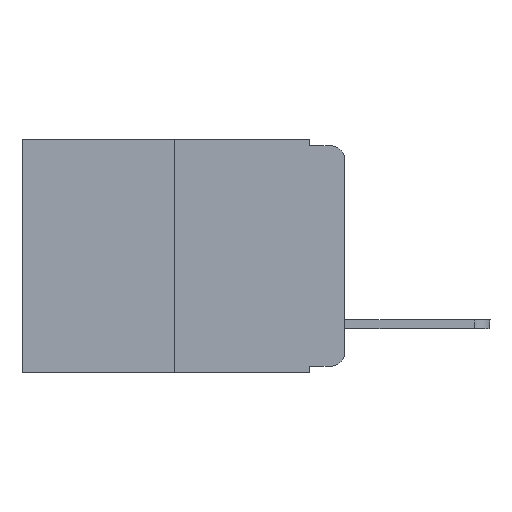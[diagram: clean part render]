
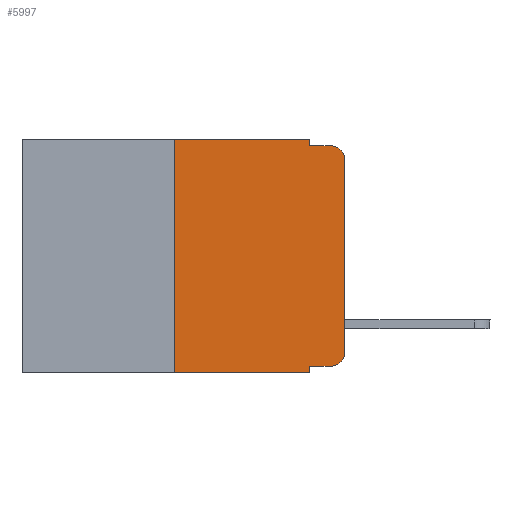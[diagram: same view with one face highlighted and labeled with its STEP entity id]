
A CAD part, left-side view. The second image highlights one B-rep face of the part: STEP entity #5997.
In plain terms, the highlighted planar face has unit normal (-1, 0, 0).
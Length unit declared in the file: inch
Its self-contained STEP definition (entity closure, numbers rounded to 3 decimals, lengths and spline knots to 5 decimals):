
#71 = EDGE_LOOP ( 'NONE', ( #4447, #2612, #941, #431, #14906, #1251, #9153, #8922, #10786, #6475 ) ) ;
#115 = LINE ( 'NONE', #4852, #1007 ) ;
#431 = ORIENTED_EDGE ( 'NONE', *, *, #6474, .F. ) ;
#554 = CARTESIAN_POINT ( 'NONE',  ( 0., 0., 0. ) ) ;
#941 = ORIENTED_EDGE ( 'NONE', *, *, #1048, .F. ) ;
#1007 = VECTOR ( 'NONE', #3630, 39.37008 ) ;
#1048 = EDGE_CURVE ( 'NONE', #14883, #9292, #13032, .T. ) ;
#1094 = VERTEX_POINT ( 'NONE', #13824 ) ;
#1161 = EDGE_CURVE ( 'NONE', #6548, #1186, #4640, .T. ) ;
#1186 = VERTEX_POINT ( 'NONE', #9371 ) ;
#1251 = ORIENTED_EDGE ( 'NONE', *, *, #9533, .F. ) ;
#1529 = VECTOR ( 'NONE', #3277, 39.37008 ) ;
#1835 = LINE ( 'NONE', #14766, #11890 ) ;
#2115 = CARTESIAN_POINT ( 'NONE',  ( 0., 0., -0.313 ) ) ;
#2176 = CARTESIAN_POINT ( 'NONE',  ( 0., 0.051, 0. ) ) ;
#2202 = DIRECTION ( 'NONE',  ( 1., 0., 0. ) ) ;
#2219 = AXIS2_PLACEMENT_3D ( 'NONE', #8562, #2857, #4014 ) ;
#2291 = CARTESIAN_POINT ( 'NONE',  ( 0., 0.051, -0.01 ) ) ;
#2612 = ORIENTED_EDGE ( 'NONE', *, *, #7987, .T. ) ;
#2713 = LINE ( 'NONE', #3019, #14389 ) ;
#2857 = DIRECTION ( 'NONE',  ( -1., 0., 0. ) ) ;
#2916 = DIRECTION ( 'NONE',  ( 0., 0., 1. ) ) ;
#3019 = CARTESIAN_POINT ( 'NONE',  ( 0., 0.473, 0. ) ) ;
#3277 = DIRECTION ( 'NONE',  ( 0., -1., 0. ) ) ;
#3625 = CARTESIAN_POINT ( 'NONE',  ( 0., 0.051, 0. ) ) ;
#3630 = DIRECTION ( 'NONE',  ( 0., 0., 1. ) ) ;
#3824 = VECTOR ( 'NONE', #15076, 39.37008 ) ;
#4014 = DIRECTION ( 'NONE',  ( 0., 0., -1. ) ) ;
#4122 = CIRCLE ( 'NONE', #5541, 0.02 ) ;
#4413 = DIRECTION ( 'NONE',  ( 0., -1., 0. ) ) ;
#4447 = ORIENTED_EDGE ( 'NONE', *, *, #13112, .T. ) ;
#4640 = LINE ( 'NONE', #10263, #1529 ) ;
#4852 = CARTESIAN_POINT ( 'NONE',  ( 0., 0.25, 0. ) ) ;
#5175 = VECTOR ( 'NONE', #4413, 39.37008 ) ;
#5195 = CARTESIAN_POINT ( 'NONE',  ( 0., 0.25, 0. ) ) ;
#5541 = AXIS2_PLACEMENT_3D ( 'NONE', #6458, #14617, #13501 ) ;
#5729 = CARTESIAN_POINT ( 'NONE',  ( 0., 0.473, -0.343 ) ) ;
#5767 = CARTESIAN_POINT ( 'NONE',  ( 0., 0.473, 0. ) ) ;
#5997 = ADVANCED_FACE ( 'NONE', ( #12350 ), #6975, .F. ) ;
#6458 = CARTESIAN_POINT ( 'NONE',  ( 0., 0.02, -0.313 ) ) ;
#6474 = EDGE_CURVE ( 'NONE', #11374, #14883, #1835, .T. ) ;
#6475 = ORIENTED_EDGE ( 'NONE', *, *, #8776, .T. ) ;
#6548 = VERTEX_POINT ( 'NONE', #14654 ) ;
#6975 = PLANE ( 'NONE',  #9630 ) ;
#7587 = DIRECTION ( 'NONE',  ( 0., 0., -1. ) ) ;
#7809 = EDGE_CURVE ( 'NONE', #1094, #10019, #7991, .T. ) ;
#7987 = EDGE_CURVE ( 'NONE', #13256, #9292, #10720, .T. ) ;
#7991 = LINE ( 'NONE', #5729, #11484 ) ;
#8155 = VERTEX_POINT ( 'NONE', #5195 ) ;
#8485 = CARTESIAN_POINT ( 'NONE',  ( 0., 0., -0.03 ) ) ;
#8562 = CARTESIAN_POINT ( 'NONE',  ( 0., 0.02, -0.03 ) ) ;
#8776 = EDGE_CURVE ( 'NONE', #1186, #10835, #4122, .T. ) ;
#8922 = ORIENTED_EDGE ( 'NONE', *, *, #12785, .F. ) ;
#9153 = ORIENTED_EDGE ( 'NONE', *, *, #7809, .T. ) ;
#9292 = VERTEX_POINT ( 'NONE', #9966 ) ;
#9371 = CARTESIAN_POINT ( 'NONE',  ( 0., 0.02, -0.333 ) ) ;
#9533 = EDGE_CURVE ( 'NONE', #1094, #8155, #115, .T. ) ;
#9630 = AXIS2_PLACEMENT_3D ( 'NONE', #5767, #2202, #12869 ) ;
#9966 = CARTESIAN_POINT ( 'NONE',  ( 0., 0.02, -0.01 ) ) ;
#10019 = VERTEX_POINT ( 'NONE', #14010 ) ;
#10263 = CARTESIAN_POINT ( 'NONE',  ( 0., 0.051, -0.333 ) ) ;
#10720 = CIRCLE ( 'NONE', #2219, 0.02 ) ;
#10751 = CARTESIAN_POINT ( 'NONE',  ( 0., 0.051, -0.01 ) ) ;
#10786 = ORIENTED_EDGE ( 'NONE', *, *, #1161, .T. ) ;
#10835 = VERTEX_POINT ( 'NONE', #2115 ) ;
#11183 = DIRECTION ( 'NONE',  ( 0., -1., 0. ) ) ;
#11374 = VERTEX_POINT ( 'NONE', #3625 ) ;
#11484 = VECTOR ( 'NONE', #15119, 39.37008 ) ;
#11890 = VECTOR ( 'NONE', #7587, 39.37008 ) ;
#12350 = FACE_OUTER_BOUND ( 'NONE', #71, .T. ) ;
#12785 = EDGE_CURVE ( 'NONE', #6548, #10019, #14781, .T. ) ;
#12869 = DIRECTION ( 'NONE',  ( 0., 0., -1. ) ) ;
#13032 = LINE ( 'NONE', #2291, #5175 ) ;
#13112 = EDGE_CURVE ( 'NONE', #10835, #13256, #13883, .T. ) ;
#13256 = VERTEX_POINT ( 'NONE', #8485 ) ;
#13501 = DIRECTION ( 'NONE',  ( 0., 0., -1. ) ) ;
#13824 = CARTESIAN_POINT ( 'NONE',  ( 0., 0.25, -0.343 ) ) ;
#13883 = LINE ( 'NONE', #554, #14961 ) ;
#13915 = EDGE_CURVE ( 'NONE', #8155, #11374, #2713, .T. ) ;
#14010 = CARTESIAN_POINT ( 'NONE',  ( 0., 0.051, -0.343 ) ) ;
#14389 = VECTOR ( 'NONE', #11183, 39.37008 ) ;
#14617 = DIRECTION ( 'NONE',  ( -1., 0., 0. ) ) ;
#14654 = CARTESIAN_POINT ( 'NONE',  ( 0., 0.051, -0.333 ) ) ;
#14766 = CARTESIAN_POINT ( 'NONE',  ( 0., 0.051, 0. ) ) ;
#14781 = LINE ( 'NONE', #2176, #3824 ) ;
#14883 = VERTEX_POINT ( 'NONE', #10751 ) ;
#14906 = ORIENTED_EDGE ( 'NONE', *, *, #13915, .F. ) ;
#14961 = VECTOR ( 'NONE', #2916, 39.37008 ) ;
#15076 = DIRECTION ( 'NONE',  ( 0., 0., -1. ) ) ;
#15119 = DIRECTION ( 'NONE',  ( 0., -1., 0. ) ) ;
